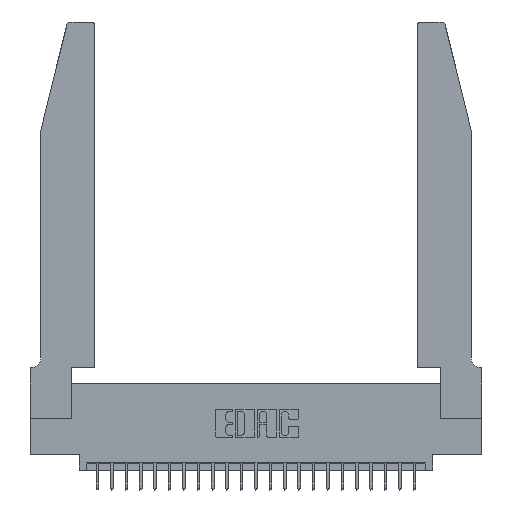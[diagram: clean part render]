
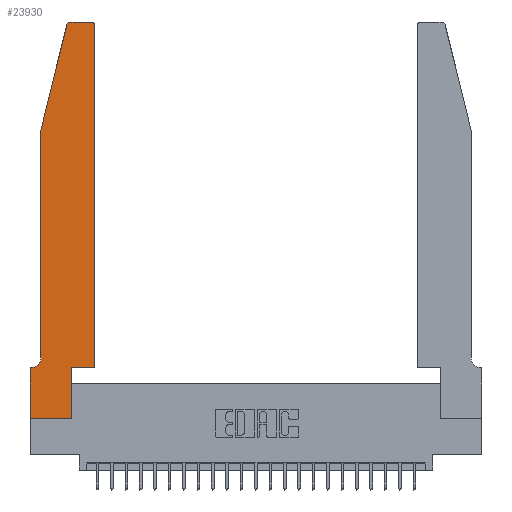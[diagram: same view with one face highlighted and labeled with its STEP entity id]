
A CAD part, top view. The second image highlights one B-rep face of the part: STEP entity #23930.
In plain terms, the highlighted planar face has unit normal (0, 0, 1).
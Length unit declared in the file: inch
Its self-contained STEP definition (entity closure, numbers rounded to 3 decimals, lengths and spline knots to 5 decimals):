
#196 = EDGE_CURVE ( 'NONE', #14136, #25162, #6199, .T. ) ;
#262 = EDGE_CURVE ( 'NONE', #21833, #12146, #20827, .T. ) ;
#265 = DIRECTION ( 'NONE',  ( 1., 0., 0. ) ) ;
#267 = AXIS2_PLACEMENT_3D ( 'NONE', #25362, #23432, #3746 ) ;
#538 = EDGE_CURVE ( 'NONE', #13470, #24453, #10751, .T. ) ;
#712 = CARTESIAN_POINT ( 'NONE',  ( 0.0755, 2., 0.37 ) ) ;
#792 = DIRECTION ( 'NONE',  ( -1., 0., 0. ) ) ;
#1332 = CARTESIAN_POINT ( 'NONE',  ( 0.2605, 2.75, 0.37 ) ) ;
#1442 = ORIENTED_EDGE ( 'NONE', *, *, #538, .T. ) ;
#1688 = EDGE_CURVE ( 'NONE', #12146, #13470, #13037, .T. ) ;
#1993 = VERTEX_POINT ( 'NONE', #3772 ) ;
#2130 = ORIENTED_EDGE ( 'NONE', *, *, #23685, .T. ) ;
#2149 = EDGE_CURVE ( 'NONE', #3372, #14411, #10458, .T. ) ;
#2484 = PLANE ( 'NONE',  #8970 ) ;
#2734 = EDGE_CURVE ( 'NONE', #14411, #14136, #5736, .T. ) ;
#2833 = CARTESIAN_POINT ( 'NONE',  ( 0.0755, 2., 0.37 ) ) ;
#3116 = EDGE_CURVE ( 'NONE', #4286, #13999, #12677, .T. ) ;
#3145 = VECTOR ( 'NONE', #20577, 39.37008 ) ;
#3200 = VECTOR ( 'NONE', #9186, 39.37008 ) ;
#3372 = VERTEX_POINT ( 'NONE', #13701 ) ;
#3475 = EDGE_CURVE ( 'NONE', #19757, #1993, #23430, .T. ) ;
#3746 = DIRECTION ( 'NONE',  ( 1., 0., 0. ) ) ;
#3772 = CARTESIAN_POINT ( 'NONE',  ( 0.25487, 2.72718, 0.37 ) ) ;
#3983 = VECTOR ( 'NONE', #15877, 39.37008 ) ;
#4154 = FACE_OUTER_BOUND ( 'NONE', #14304, .T. ) ;
#4286 = VERTEX_POINT ( 'NONE', #10638 ) ;
#4294 = DIRECTION ( 'NONE',  ( 0., 0., -1. ) ) ;
#5174 = AXIS2_PLACEMENT_3D ( 'NONE', #18173, #4294, #10124 ) ;
#5736 = LINE ( 'NONE', #13508, #13892 ) ;
#6199 = LINE ( 'NONE', #14483, #14215 ) ;
#6311 = DIRECTION ( 'NONE',  ( -0.239, -0.971, 0. ) ) ;
#6845 = VECTOR ( 'NONE', #19626, 39.37008 ) ;
#7200 = CARTESIAN_POINT ( 'NONE',  ( 0.284, 2.75, 0.37 ) ) ;
#7463 = ORIENTED_EDGE ( 'NONE', *, *, #2149, .T. ) ;
#7797 = CARTESIAN_POINT ( 'NONE',  ( 0., 0., 0.37 ) ) ;
#8970 = AXIS2_PLACEMENT_3D ( 'NONE', #18002, #10360, #265 ) ;
#9127 = CARTESIAN_POINT ( 'NONE',  ( 0.0755, 0.42, 0.37 ) ) ;
#9186 = DIRECTION ( 'NONE',  ( -1., 0., 0. ) ) ;
#9241 = ORIENTED_EDGE ( 'NONE', *, *, #262, .T. ) ;
#9274 = EDGE_CURVE ( 'NONE', #24453, #3372, #11846, .T. ) ;
#9529 = ORIENTED_EDGE ( 'NONE', *, *, #1688, .T. ) ;
#10124 = DIRECTION ( 'NONE',  ( -1., 0., 0. ) ) ;
#10360 = DIRECTION ( 'NONE',  ( 0., 0., 1. ) ) ;
#10458 = LINE ( 'NONE', #13990, #3145 ) ;
#10478 = CARTESIAN_POINT ( 'NONE',  ( 0.0755, 0.35, 0.37 ) ) ;
#10638 = CARTESIAN_POINT ( 'NONE',  ( 0.4505, 2.72, 0.37 ) ) ;
#10751 = LINE ( 'NONE', #10478, #15066 ) ;
#10865 = CARTESIAN_POINT ( 'NONE',  ( 0.0755, 2., 0.37 ) ) ;
#10943 = VECTOR ( 'NONE', #24718, 39.37008 ) ;
#11368 = ORIENTED_EDGE ( 'NONE', *, *, #196, .T. ) ;
#11440 = VECTOR ( 'NONE', #6311, 39.37008 ) ;
#11631 = CARTESIAN_POINT ( 'NONE',  ( 0.4205, 2.75, 0.37 ) ) ;
#11826 = EDGE_CURVE ( 'NONE', #25162, #4286, #17579, .T. ) ;
#11846 = LINE ( 'NONE', #7797, #6845 ) ;
#12024 = CARTESIAN_POINT ( 'NONE',  ( 0.2865, 0.35, 0.37 ) ) ;
#12049 = EDGE_CURVE ( 'NONE', #1993, #21833, #24317, .T. ) ;
#12146 = VERTEX_POINT ( 'NONE', #9127 ) ;
#12189 = DIRECTION ( 'NONE',  ( 1., 0., 0. ) ) ;
#12273 = AXIS2_PLACEMENT_3D ( 'NONE', #24494, #12458, #12189 ) ;
#12458 = DIRECTION ( 'NONE',  ( 0., 0., 1. ) ) ;
#12677 = CIRCLE ( 'NONE', #12273, 0.03 ) ;
#12797 = CARTESIAN_POINT ( 'NONE',  ( 0., 0.35, 0.37 ) ) ;
#13037 = CIRCLE ( 'NONE', #5174, 0.07 ) ;
#13470 = VERTEX_POINT ( 'NONE', #22945 ) ;
#13508 = CARTESIAN_POINT ( 'NONE',  ( 0.2865, 0.35, 0.37 ) ) ;
#13701 = CARTESIAN_POINT ( 'NONE',  ( 0., 0., 0.37 ) ) ;
#13753 = ORIENTED_EDGE ( 'NONE', *, *, #2734, .T. ) ;
#13892 = VECTOR ( 'NONE', #21813, 39.37008 ) ;
#13990 = CARTESIAN_POINT ( 'NONE',  ( 0., 0., 0.37 ) ) ;
#13997 = CARTESIAN_POINT ( 'NONE',  ( 0.4505, 0.35, 0.37 ) ) ;
#13999 = VERTEX_POINT ( 'NONE', #11631 ) ;
#14136 = VERTEX_POINT ( 'NONE', #12024 ) ;
#14215 = VECTOR ( 'NONE', #18252, 39.37008 ) ;
#14304 = EDGE_LOOP ( 'NONE', ( #2130, #15881, #23176, #9241, #9529, #1442, #15865, #7463, #13753, #11368, #16231, #23887 ) ) ;
#14411 = VERTEX_POINT ( 'NONE', #24822 ) ;
#14483 = CARTESIAN_POINT ( 'NONE',  ( 0.4505, 0.35, 0.37 ) ) ;
#15066 = VECTOR ( 'NONE', #792, 39.37008 ) ;
#15865 = ORIENTED_EDGE ( 'NONE', *, *, #9274, .T. ) ;
#15877 = DIRECTION ( 'NONE',  ( 0., 1., 0. ) ) ;
#15881 = ORIENTED_EDGE ( 'NONE', *, *, #3475, .T. ) ;
#16231 = ORIENTED_EDGE ( 'NONE', *, *, #11826, .T. ) ;
#17579 = LINE ( 'NONE', #19546, #3983 ) ;
#18002 = CARTESIAN_POINT ( 'NONE',  ( 0., 0.35, 0.37 ) ) ;
#18173 = CARTESIAN_POINT ( 'NONE',  ( 0.0055, 0.42, 0.37 ) ) ;
#18252 = DIRECTION ( 'NONE',  ( 1., 0., 0. ) ) ;
#19076 = LINE ( 'NONE', #1332, #3200 ) ;
#19546 = CARTESIAN_POINT ( 'NONE',  ( 0.4505, 0.35, 0.37 ) ) ;
#19626 = DIRECTION ( 'NONE',  ( 0., -1., 0. ) ) ;
#19757 = VERTEX_POINT ( 'NONE', #7200 ) ;
#20577 = DIRECTION ( 'NONE',  ( 1., 0., 0. ) ) ;
#20827 = LINE ( 'NONE', #10865, #10943 ) ;
#21813 = DIRECTION ( 'NONE',  ( 0., 1., 0. ) ) ;
#21833 = VERTEX_POINT ( 'NONE', #712 ) ;
#22945 = CARTESIAN_POINT ( 'NONE',  ( 0.0055, 0.35, 0.37 ) ) ;
#23176 = ORIENTED_EDGE ( 'NONE', *, *, #12049, .T. ) ;
#23430 = CIRCLE ( 'NONE', #267, 0.03 ) ;
#23432 = DIRECTION ( 'NONE',  ( 0., 0., 1. ) ) ;
#23685 = EDGE_CURVE ( 'NONE', #13999, #19757, #19076, .T. ) ;
#23887 = ORIENTED_EDGE ( 'NONE', *, *, #3116, .T. ) ;
#23930 = ADVANCED_FACE ( 'NONE', ( #4154 ), #2484, .T. ) ;
#24317 = LINE ( 'NONE', #2833, #11440 ) ;
#24453 = VERTEX_POINT ( 'NONE', #12797 ) ;
#24494 = CARTESIAN_POINT ( 'NONE',  ( 0.4205, 2.72, 0.37 ) ) ;
#24718 = DIRECTION ( 'NONE',  ( 0., -1., 0. ) ) ;
#24822 = CARTESIAN_POINT ( 'NONE',  ( 0.2865, 0., 0.37 ) ) ;
#25162 = VERTEX_POINT ( 'NONE', #13997 ) ;
#25362 = CARTESIAN_POINT ( 'NONE',  ( 0.284, 2.72, 0.37 ) ) ;
